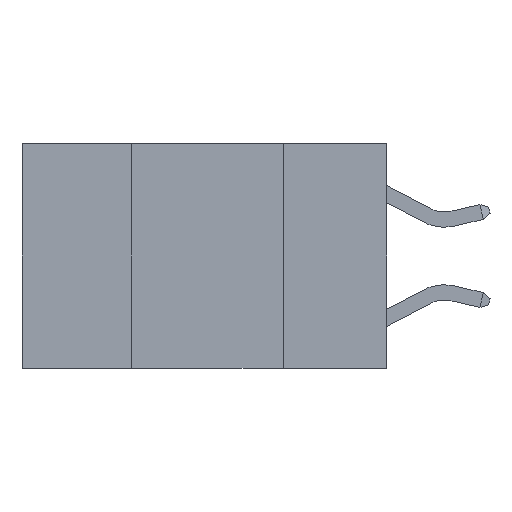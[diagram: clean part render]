
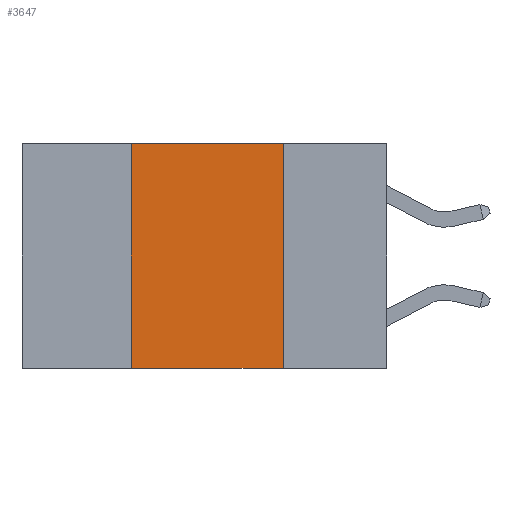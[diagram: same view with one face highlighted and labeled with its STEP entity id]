
A CAD part, left-side view. The second image highlights one B-rep face of the part: STEP entity #3647.
In plain terms, the highlighted planar face has unit normal (-1, 0, 0).
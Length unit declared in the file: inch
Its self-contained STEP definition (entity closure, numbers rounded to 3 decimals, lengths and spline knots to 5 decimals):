
#88 = DIRECTION ( 'NONE',  ( 1., 0., 0. ) ) ;
#106 = VECTOR ( 'NONE', #11724, 39.37008 ) ;
#160 = CARTESIAN_POINT ( 'NONE',  ( 0., 0.17, 0. ) ) ;
#264 = CARTESIAN_POINT ( 'NONE',  ( 0., 0.17, 0. ) ) ;
#1713 = CARTESIAN_POINT ( 'NONE',  ( 0., 0.6, -0.37 ) ) ;
#1812 = VECTOR ( 'NONE', #13879, 39.37008 ) ;
#2170 = EDGE_CURVE ( 'NONE', #8471, #6058, #10268, .T. ) ;
#2297 = EDGE_LOOP ( 'NONE', ( #6129, #12242, #18416, #12070 ) ) ;
#3342 = CARTESIAN_POINT ( 'NONE',  ( 0., 0.6, 0. ) ) ;
#3647 = ADVANCED_FACE ( 'NONE', ( #13254 ), #9012, .F. ) ;
#4118 = VECTOR ( 'NONE', #15817, 39.37008 ) ;
#5790 = EDGE_CURVE ( 'NONE', #8471, #7240, #17244, .T. ) ;
#5985 = AXIS2_PLACEMENT_3D ( 'NONE', #3342, #88, #7685 ) ;
#6058 = VERTEX_POINT ( 'NONE', #12354 ) ;
#6129 = ORIENTED_EDGE ( 'NONE', *, *, #18071, .F. ) ;
#7240 = VERTEX_POINT ( 'NONE', #12560 ) ;
#7685 = DIRECTION ( 'NONE',  ( 0., 0., -1. ) ) ;
#8415 = VERTEX_POINT ( 'NONE', #160 ) ;
#8471 = VERTEX_POINT ( 'NONE', #11907 ) ;
#9012 = PLANE ( 'NONE',  #5985 ) ;
#9886 = VECTOR ( 'NONE', #16126, 39.37008 ) ;
#10268 = LINE ( 'NONE', #1713, #106 ) ;
#10362 = LINE ( 'NONE', #264, #9886 ) ;
#10912 = LINE ( 'NONE', #16764, #1812 ) ;
#11724 = DIRECTION ( 'NONE',  ( 0., -1., 0. ) ) ;
#11907 = CARTESIAN_POINT ( 'NONE',  ( 0., 0.42, -0.37 ) ) ;
#12070 = ORIENTED_EDGE ( 'NONE', *, *, #2170, .T. ) ;
#12242 = ORIENTED_EDGE ( 'NONE', *, *, #15612, .F. ) ;
#12354 = CARTESIAN_POINT ( 'NONE',  ( 0., 0.17, -0.37 ) ) ;
#12560 = CARTESIAN_POINT ( 'NONE',  ( 0., 0.42, 0. ) ) ;
#13254 = FACE_OUTER_BOUND ( 'NONE', #2297, .T. ) ;
#13879 = DIRECTION ( 'NONE',  ( 0., -1., 0. ) ) ;
#15612 = EDGE_CURVE ( 'NONE', #7240, #8415, #10912, .T. ) ;
#15817 = DIRECTION ( 'NONE',  ( 0., 0., 1. ) ) ;
#15911 = CARTESIAN_POINT ( 'NONE',  ( 0., 0.42, 0. ) ) ;
#16126 = DIRECTION ( 'NONE',  ( 0., 0., -1. ) ) ;
#16764 = CARTESIAN_POINT ( 'NONE',  ( 0., 0.6, 0. ) ) ;
#17244 = LINE ( 'NONE', #15911, #4118 ) ;
#18071 = EDGE_CURVE ( 'NONE', #8415, #6058, #10362, .T. ) ;
#18416 = ORIENTED_EDGE ( 'NONE', *, *, #5790, .F. ) ;
